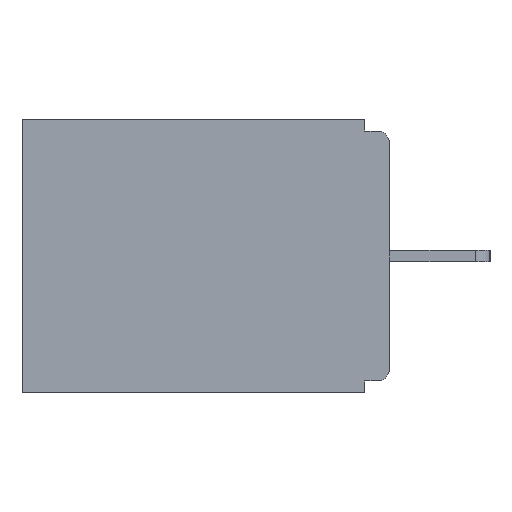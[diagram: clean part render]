
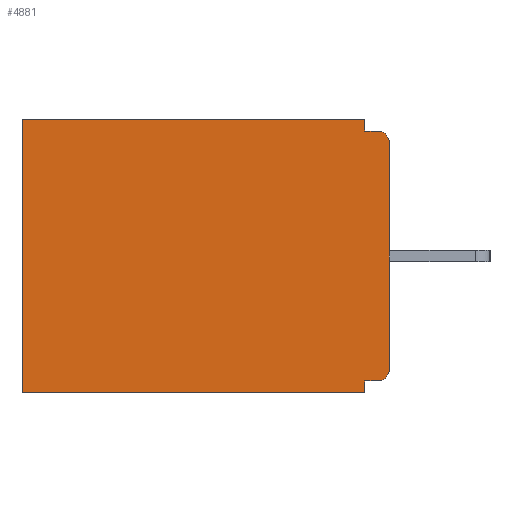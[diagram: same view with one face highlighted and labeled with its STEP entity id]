
A CAD part, left-side view. The second image highlights one B-rep face of the part: STEP entity #4881.
In plain terms, the highlighted planar face has unit normal (-1, 0, 0).
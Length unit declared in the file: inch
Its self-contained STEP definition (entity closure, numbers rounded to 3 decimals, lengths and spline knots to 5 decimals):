
#60 = VECTOR ( 'NONE', #7456, 39.37008 ) ;
#365 = CARTESIAN_POINT ( 'NONE',  ( 0.298, 0., -0.328 ) ) ;
#457 = VERTEX_POINT ( 'NONE', #6377 ) ;
#740 = EDGE_CURVE ( 'NONE', #13775, #13689, #13259, .T. ) ;
#973 = CARTESIAN_POINT ( 'NONE',  ( 0.298, 0.031, 0. ) ) ;
#985 = DIRECTION ( 'NONE',  ( -1., 0., 0. ) ) ;
#1032 = EDGE_CURVE ( 'NONE', #6658, #12709, #13712, .T. ) ;
#1464 = EDGE_CURVE ( 'NONE', #4744, #457, #2612, .T. ) ;
#1551 = DIRECTION ( 'NONE',  ( 0., -1., 0. ) ) ;
#1675 = LINE ( 'NONE', #7423, #12568 ) ;
#1966 = ORIENTED_EDGE ( 'NONE', *, *, #14756, .F. ) ;
#2003 = CARTESIAN_POINT ( 'NONE',  ( 0.298, 0., -0.313 ) ) ;
#2612 = LINE ( 'NONE', #5074, #9265 ) ;
#2628 = CARTESIAN_POINT ( 'NONE',  ( 0.298, 0.015, -0.015 ) ) ;
#2686 = AXIS2_PLACEMENT_3D ( 'NONE', #13426, #6412, #4130 ) ;
#2881 = CARTESIAN_POINT ( 'NONE',  ( 0.298, 0., -0.03 ) ) ;
#2909 = LINE ( 'NONE', #7675, #60 ) ;
#3220 = ORIENTED_EDGE ( 'NONE', *, *, #13934, .T. ) ;
#3288 = ORIENTED_EDGE ( 'NONE', *, *, #4747, .F. ) ;
#3758 = DIRECTION ( 'NONE',  ( 0., 1., 0. ) ) ;
#4049 = CARTESIAN_POINT ( 'NONE',  ( 0.298, 0., 0. ) ) ;
#4130 = DIRECTION ( 'NONE',  ( 0., 0., -1. ) ) ;
#4141 = DIRECTION ( 'NONE',  ( 0., 0., -1. ) ) ;
#4604 = ORIENTED_EDGE ( 'NONE', *, *, #740, .F. ) ;
#4744 = VERTEX_POINT ( 'NONE', #7167 ) ;
#4747 = EDGE_CURVE ( 'NONE', #14720, #12709, #10665, .T. ) ;
#4881 = ADVANCED_FACE ( 'NONE', ( #5463 ), #12247, .F. ) ;
#5007 = CARTESIAN_POINT ( 'NONE',  ( 0.298, 0., -0.015 ) ) ;
#5074 = CARTESIAN_POINT ( 'NONE',  ( 0.298, 0.46, 0. ) ) ;
#5348 = EDGE_CURVE ( 'NONE', #12022, #457, #2909, .T. ) ;
#5370 = VECTOR ( 'NONE', #1551, 39.37008 ) ;
#5463 = FACE_OUTER_BOUND ( 'NONE', #14041, .T. ) ;
#5896 = CARTESIAN_POINT ( 'NONE',  ( 0.298, 0.031, -0.015 ) ) ;
#6286 = DIRECTION ( 'NONE',  ( 0., 0., -1. ) ) ;
#6377 = CARTESIAN_POINT ( 'NONE',  ( 0.298, 0.46, -0.343 ) ) ;
#6412 = DIRECTION ( 'NONE',  ( 1., 0., 0. ) ) ;
#6592 = ORIENTED_EDGE ( 'NONE', *, *, #1464, .T. ) ;
#6658 = VERTEX_POINT ( 'NONE', #11443 ) ;
#6812 = VERTEX_POINT ( 'NONE', #973 ) ;
#7167 = CARTESIAN_POINT ( 'NONE',  ( 0.298, 0.46, 0. ) ) ;
#7272 = AXIS2_PLACEMENT_3D ( 'NONE', #10541, #12100, #12021 ) ;
#7423 = CARTESIAN_POINT ( 'NONE',  ( 0.298, 0.031, -0.343 ) ) ;
#7456 = DIRECTION ( 'NONE',  ( 0., 1., 0. ) ) ;
#7530 = CARTESIAN_POINT ( 'NONE',  ( 0.298, 0.031, -0.328 ) ) ;
#7580 = VECTOR ( 'NONE', #8719, 39.37008 ) ;
#7675 = CARTESIAN_POINT ( 'NONE',  ( 0.298, 0., -0.343 ) ) ;
#7848 = VECTOR ( 'NONE', #4141, 39.37008 ) ;
#8366 = CARTESIAN_POINT ( 'NONE',  ( 0.298, 0., 0. ) ) ;
#8420 = DIRECTION ( 'NONE',  ( 0., 0., -1. ) ) ;
#8590 = VECTOR ( 'NONE', #3758, 39.37008 ) ;
#8686 = CARTESIAN_POINT ( 'NONE',  ( 0.298, 0.031, -0.343 ) ) ;
#8719 = DIRECTION ( 'NONE',  ( 0., 1., 0. ) ) ;
#8832 = AXIS2_PLACEMENT_3D ( 'NONE', #11139, #985, #9945 ) ;
#9265 = VECTOR ( 'NONE', #8420, 39.37008 ) ;
#9613 = EDGE_CURVE ( 'NONE', #14720, #13689, #11224, .T. ) ;
#9785 = CARTESIAN_POINT ( 'NONE',  ( 0.298, 0.031, -0.343 ) ) ;
#9875 = VERTEX_POINT ( 'NONE', #7530 ) ;
#9945 = DIRECTION ( 'NONE',  ( 0., 0., -1. ) ) ;
#10375 = LINE ( 'NONE', #365, #8590 ) ;
#10398 = ORIENTED_EDGE ( 'NONE', *, *, #1032, .T. ) ;
#10541 = CARTESIAN_POINT ( 'NONE',  ( 0.298, 0.015, -0.313 ) ) ;
#10560 = VECTOR ( 'NONE', #11712, 39.37008 ) ;
#10665 = LINE ( 'NONE', #8366, #10560 ) ;
#10895 = LINE ( 'NONE', #9785, #7848 ) ;
#11139 = CARTESIAN_POINT ( 'NONE',  ( 0.298, 0.015, -0.03 ) ) ;
#11145 = ORIENTED_EDGE ( 'NONE', *, *, #9613, .T. ) ;
#11224 = CIRCLE ( 'NONE', #8832, 0.015 ) ;
#11443 = CARTESIAN_POINT ( 'NONE',  ( 0.298, 0.015, -0.328 ) ) ;
#11526 = EDGE_CURVE ( 'NONE', #6658, #9875, #10375, .T. ) ;
#11712 = DIRECTION ( 'NONE',  ( 0., 0., -1. ) ) ;
#11883 = ORIENTED_EDGE ( 'NONE', *, *, #11526, .F. ) ;
#12021 = DIRECTION ( 'NONE',  ( 0., 0., -1. ) ) ;
#12022 = VERTEX_POINT ( 'NONE', #8686 ) ;
#12100 = DIRECTION ( 'NONE',  ( -1., 0., 0. ) ) ;
#12247 = PLANE ( 'NONE',  #2686 ) ;
#12332 = ORIENTED_EDGE ( 'NONE', *, *, #13477, .F. ) ;
#12568 = VECTOR ( 'NONE', #6286, 39.37008 ) ;
#12709 = VERTEX_POINT ( 'NONE', #2003 ) ;
#13259 = LINE ( 'NONE', #5007, #5370 ) ;
#13426 = CARTESIAN_POINT ( 'NONE',  ( 0.298, 0., 0. ) ) ;
#13477 = EDGE_CURVE ( 'NONE', #6812, #13775, #10895, .T. ) ;
#13689 = VERTEX_POINT ( 'NONE', #2628 ) ;
#13712 = CIRCLE ( 'NONE', #7272, 0.015 ) ;
#13775 = VERTEX_POINT ( 'NONE', #5896 ) ;
#13934 = EDGE_CURVE ( 'NONE', #6812, #4744, #14240, .T. ) ;
#14041 = EDGE_LOOP ( 'NONE', ( #11145, #4604, #12332, #3220, #6592, #14738, #1966, #11883, #10398, #3288 ) ) ;
#14240 = LINE ( 'NONE', #4049, #7580 ) ;
#14720 = VERTEX_POINT ( 'NONE', #2881 ) ;
#14738 = ORIENTED_EDGE ( 'NONE', *, *, #5348, .F. ) ;
#14756 = EDGE_CURVE ( 'NONE', #9875, #12022, #1675, .T. ) ;
